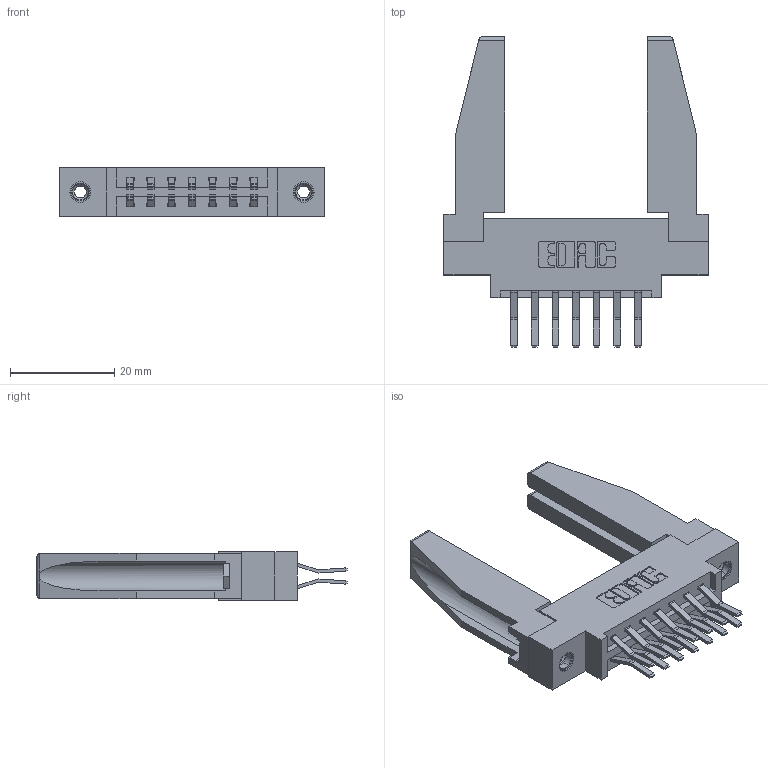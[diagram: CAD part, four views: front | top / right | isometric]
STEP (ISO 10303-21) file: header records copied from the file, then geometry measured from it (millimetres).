
FILE_DESCRIPTION (( 'STEP AP203' ), '1' );
FILE_NAME ('337-014-560-878.STEP', '2019-10-10T17:34:28', ( '' ), ( '' ), 'SwSTEP 2.0', 'SolidWorks 2016', '' );
FILE_SCHEMA (( 'CONFIG_CONTROL_DESIGN' ));
Length unit declared in the file: inch
Products named in the file (5): 345-292-001_560 Tail; 337-014-560-878; 345-250-001_345-250-001-102; 337 Part_0.170 Offset - 0.156 Dia-TI; 307-220-078
Assembly tree (19 placements, depth 2):
  337-014-560-878
    337 Part_0.170 Offset - 0.156 Dia-TI
    345-292-001_560 Tail  x14
    345-250-001_345-250-001-102  x2
    307-220-078  x2
Bounding box: 50.75 x 59.58 x 9.4 mm (x, y, z)
Volume: 8850.1 mm3; surface area: 9354.4 mm2
Topology: 19 solids, 19 shells, 1032 faces, 2991 edges, 1966 vertices
Faces by surface type: plane 690, cylinder 326, cone 12, torus 4
Entity records: 12614 total; most frequent: CARTESIAN_POINT 2156, ORIENTED_EDGE 2048, DIRECTION 1908, EDGE_CURVE 1024, LINE 854, VECTOR 854, VERTEX_POINT 676, AXIS2_PLACEMENT_3D 527
